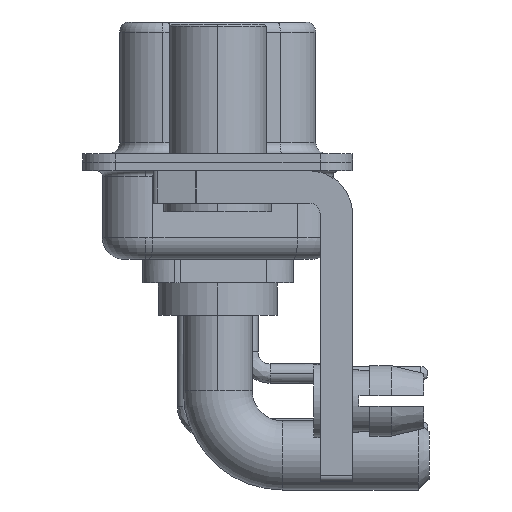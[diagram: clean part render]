
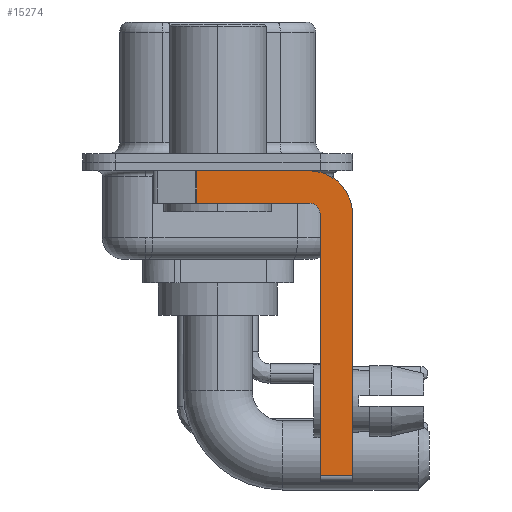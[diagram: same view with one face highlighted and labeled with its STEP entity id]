
A CAD part, left-side view. The second image highlights one B-rep face of the part: STEP entity #15274.
In plain terms, the highlighted planar face has unit normal (-1, 0, 0).
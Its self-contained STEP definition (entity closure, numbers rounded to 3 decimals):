
#427 = EDGE_CURVE ( 'NONE', #2256, #10687, #11638, .T. ) ;
#867 = LINE ( 'NONE', #5380, #19612 ) ;
#1539 = DIRECTION ( 'NONE',  ( 0., 0., -1. ) ) ;
#1808 = ORIENTED_EDGE ( 'NONE', *, *, #22795, .T. ) ;
#2256 = VERTEX_POINT ( 'NONE', #7647 ) ;
#2981 = AXIS2_PLACEMENT_3D ( 'NONE', #14254, #18502, #12349 ) ;
#3304 = FACE_OUTER_BOUND ( 'NONE', #19523, .T. ) ;
#3322 = CARTESIAN_POINT ( 'NONE',  ( -2.9, 0.978, -1.9 ) ) ;
#4233 = CARTESIAN_POINT ( 'NONE',  ( -2.9, -4.75, -2.4 ) ) ;
#4265 = CARTESIAN_POINT ( 'NONE',  ( -2.9, -4.25, -1.9 ) ) ;
#4466 = EDGE_CURVE ( 'NONE', #9325, #10303, #6682, .T. ) ;
#4651 = VERTEX_POINT ( 'NONE', #9999 ) ;
#4687 = EDGE_CURVE ( 'NONE', #4651, #2256, #25821, .T. ) ;
#4729 = CARTESIAN_POINT ( 'NONE',  ( -2.9, -6.25, -14.55 ) ) ;
#4850 = EDGE_CURVE ( 'NONE', #8625, #18827, #22593, .T. ) ;
#5380 = CARTESIAN_POINT ( 'NONE',  ( -2.9, -4.75, -14.8 ) ) ;
#5416 = CARTESIAN_POINT ( 'NONE',  ( -2.9, -4.25, -14.55 ) ) ;
#5925 = EDGE_CURVE ( 'NONE', #18827, #10303, #17587, .T. ) ;
#6331 = DIRECTION ( 'NONE',  ( 0., 1., 0. ) ) ;
#6682 = LINE ( 'NONE', #24658, #22110 ) ;
#7509 = VECTOR ( 'NONE', #20613, 1000. ) ;
#7647 = CARTESIAN_POINT ( 'NONE',  ( -2.9, -6.25, -2.4 ) ) ;
#8041 = LINE ( 'NONE', #5416, #22857 ) ;
#8206 = CARTESIAN_POINT ( 'NONE',  ( -2.9, -4.25, -1.9 ) ) ;
#8251 = ORIENTED_EDGE ( 'NONE', *, *, #23407, .F. ) ;
#8409 = DIRECTION ( 'NONE',  ( -1., 0., 0. ) ) ;
#8625 = VERTEX_POINT ( 'NONE', #4233 ) ;
#9325 = VERTEX_POINT ( 'NONE', #13947 ) ;
#9887 = CARTESIAN_POINT ( 'NONE',  ( -2.9, -4.25, -2.4 ) ) ;
#9999 = CARTESIAN_POINT ( 'NONE',  ( -2.9, -4.25, -0.4 ) ) ;
#10303 = VERTEX_POINT ( 'NONE', #3322 ) ;
#10598 = CARTESIAN_POINT ( 'NONE',  ( -2.9, -4.25, -2.4 ) ) ;
#10687 = VERTEX_POINT ( 'NONE', #4729 ) ;
#11638 = LINE ( 'NONE', #27264, #18077 ) ;
#12349 = DIRECTION ( 'NONE',  ( 0., 0., -1. ) ) ;
#13947 = CARTESIAN_POINT ( 'NONE',  ( -2.9, 0.978, -0.4 ) ) ;
#14254 = CARTESIAN_POINT ( 'NONE',  ( -2.9, -4.25, -2.4 ) ) ;
#15274 = ADVANCED_FACE ( 'NONE', ( #3304 ), #21009, .F. ) ;
#15365 = CARTESIAN_POINT ( 'NONE',  ( -2.9, -4.75, -14.55 ) ) ;
#16579 = VECTOR ( 'NONE', #6331, 1000. ) ;
#16917 = AXIS2_PLACEMENT_3D ( 'NONE', #9887, #25248, #27572 ) ;
#17587 = LINE ( 'NONE', #4265, #16579 ) ;
#17933 = AXIS2_PLACEMENT_3D ( 'NONE', #10598, #8409, #19512 ) ;
#18077 = VECTOR ( 'NONE', #1539, 1000. ) ;
#18245 = VERTEX_POINT ( 'NONE', #15365 ) ;
#18377 = ORIENTED_EDGE ( 'NONE', *, *, #24631, .F. ) ;
#18502 = DIRECTION ( 'NONE',  ( 1., 0., 0. ) ) ;
#18827 = VERTEX_POINT ( 'NONE', #8206 ) ;
#19043 = ORIENTED_EDGE ( 'NONE', *, *, #4466, .T. ) ;
#19188 = ORIENTED_EDGE ( 'NONE', *, *, #5925, .F. ) ;
#19512 = DIRECTION ( 'NONE',  ( 0., 0., 1. ) ) ;
#19523 = EDGE_LOOP ( 'NONE', ( #18377, #19043, #19188, #26359, #8251, #1808, #20440, #22794 ) ) ;
#19612 = VECTOR ( 'NONE', #27595, 1000. ) ;
#20440 = ORIENTED_EDGE ( 'NONE', *, *, #427, .F. ) ;
#20613 = DIRECTION ( 'NONE',  ( 0., -1., 0. ) ) ;
#20928 = DIRECTION ( 'NONE',  ( 0., -1., 0. ) ) ;
#21009 = PLANE ( 'NONE',  #16917 ) ;
#22110 = VECTOR ( 'NONE', #26838, 1000. ) ;
#22593 = CIRCLE ( 'NONE', #17933, 0.5 ) ;
#22794 = ORIENTED_EDGE ( 'NONE', *, *, #4687, .F. ) ;
#22795 = EDGE_CURVE ( 'NONE', #18245, #10687, #8041, .T. ) ;
#22816 = CARTESIAN_POINT ( 'NONE',  ( -2.9, 3., -0.4 ) ) ;
#22857 = VECTOR ( 'NONE', #20928, 1000. ) ;
#23407 = EDGE_CURVE ( 'NONE', #18245, #8625, #867, .T. ) ;
#24631 = EDGE_CURVE ( 'NONE', #9325, #4651, #26894, .T. ) ;
#24658 = CARTESIAN_POINT ( 'NONE',  ( -2.9, 0.978, -1.9 ) ) ;
#25248 = DIRECTION ( 'NONE',  ( 1., 0., 0. ) ) ;
#25821 = CIRCLE ( 'NONE', #2981, 2. ) ;
#26359 = ORIENTED_EDGE ( 'NONE', *, *, #4850, .F. ) ;
#26838 = DIRECTION ( 'NONE',  ( 0., 0., -1. ) ) ;
#26894 = LINE ( 'NONE', #22816, #7509 ) ;
#27264 = CARTESIAN_POINT ( 'NONE',  ( -2.9, -6.25, -2.4 ) ) ;
#27572 = DIRECTION ( 'NONE',  ( 0., 0., -1. ) ) ;
#27595 = DIRECTION ( 'NONE',  ( 0., 0., 1. ) ) ;
